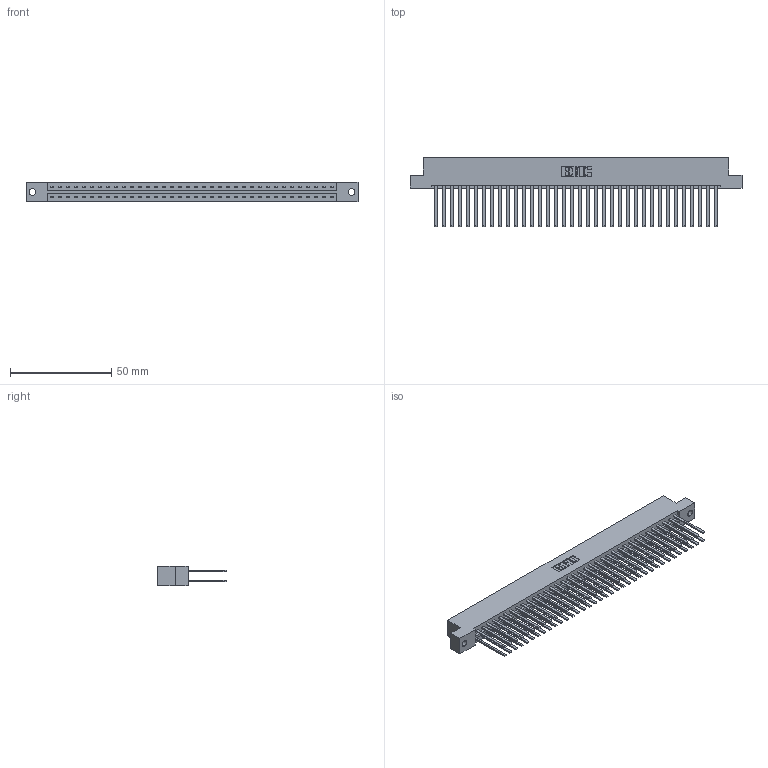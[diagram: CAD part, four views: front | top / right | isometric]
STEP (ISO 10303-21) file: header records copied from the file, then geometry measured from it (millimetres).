
FILE_DESCRIPTION (( 'STEP AP203' ), '1' );
FILE_NAME ('833-072-544-202.STEP', '2020-06-05T14:33:46', ( '' ), ( '' ), 'SwSTEP 2.0', 'SolidWorks 2020', '' );
FILE_SCHEMA (( 'CONFIG_CONTROL_DESIGN' ));
Length unit declared in the file: inch
Products named in the file (3): 345-292-001_345-293-144; 833 Part_Flush - .128 Dia; 833-072-544-202
Assembly tree (73 placements, depth 2):
  833-072-544-202
    833 Part_Flush - .128 Dia
    345-292-001_345-293-144  x72
Bounding box: 164.19 x 34.3 x 9.4 mm (x, y, z)
Volume: 17678.9 mm3; surface area: 23812.8 mm2
Topology: 73 solids, 73 shells, 3426 faces, 10175 edges, 6686 vertices
Faces by surface type: plane 2374, cylinder 1052
Entity records: 23755 total; most frequent: CARTESIAN_POINT 3942, ORIENTED_EDGE 3878, DIRECTION 3375, EDGE_CURVE 1939, LINE 1815, VECTOR 1815, VERTEX_POINT 1290, AXIS2_PLACEMENT_3D 780
